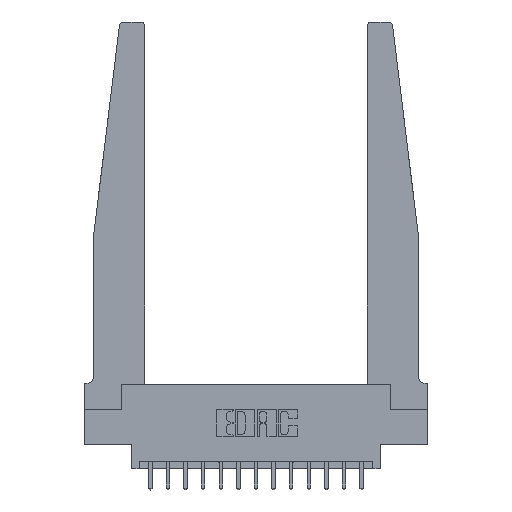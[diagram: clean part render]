
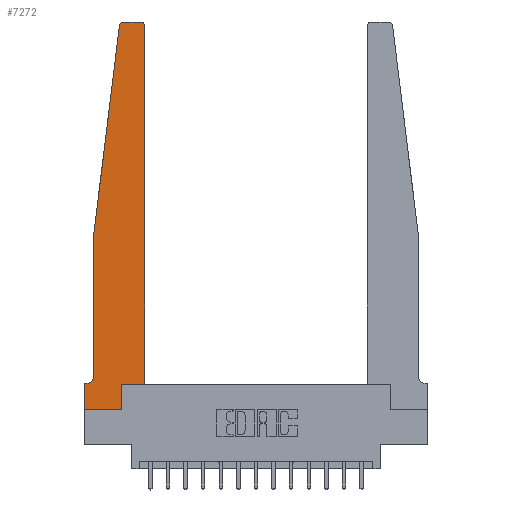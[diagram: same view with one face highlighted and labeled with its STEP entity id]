
A CAD part, top view. The second image highlights one B-rep face of the part: STEP entity #7272.
In plain terms, the highlighted planar face has unit normal (0, 0, 1).
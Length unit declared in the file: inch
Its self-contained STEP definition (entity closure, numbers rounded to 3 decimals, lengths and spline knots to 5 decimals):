
#203 = DIRECTION ( 'NONE',  ( 0., 1., 0. ) ) ;
#871 = CARTESIAN_POINT ( 'NONE',  ( 0.395, 2.75, 0.37 ) ) ;
#1552 = AXIS2_PLACEMENT_3D ( 'NONE', #4527, #13935, #5878 ) ;
#1663 = DIRECTION ( 'NONE',  ( 0., 0., 1. ) ) ;
#1771 = CARTESIAN_POINT ( 'NONE',  ( 0.065, 0.1875, 0.37 ) ) ;
#2200 = CARTESIAN_POINT ( 'NONE',  ( 0.065, 1.25, 0.37 ) ) ;
#2266 = ORIENTED_EDGE ( 'NONE', *, *, #3046, .T. ) ;
#2368 = VERTEX_POINT ( 'NONE', #9925 ) ;
#2550 = LINE ( 'NONE', #16554, #9312 ) ;
#2705 = CIRCLE ( 'NONE', #4445, 0.03 ) ;
#2726 = DIRECTION ( 'NONE',  ( 1., 0., 0. ) ) ;
#2876 = CARTESIAN_POINT ( 'NONE',  ( 0.425, 2.72, 0.37 ) ) ;
#3022 = VERTEX_POINT ( 'NONE', #5765 ) ;
#3046 = EDGE_CURVE ( 'NONE', #10043, #12302, #9291, .T. ) ;
#3104 = DIRECTION ( 'NONE',  ( -1., 0., 0. ) ) ;
#3427 = EDGE_CURVE ( 'NONE', #2368, #12764, #3769, .T. ) ;
#3631 = EDGE_CURVE ( 'NONE', #12302, #16082, #4388, .T. ) ;
#3719 = EDGE_CURVE ( 'NONE', #3022, #17066, #2705, .T. ) ;
#3769 = LINE ( 'NONE', #13399, #14915 ) ;
#3974 = VECTOR ( 'NONE', #3104, 39.37008 ) ;
#3977 = CARTESIAN_POINT ( 'NONE',  ( 0.24675, 2.72367, 0.37 ) ) ;
#4288 = FACE_OUTER_BOUND ( 'NONE', #10441, .T. ) ;
#4388 = LINE ( 'NONE', #1771, #3974 ) ;
#4445 = AXIS2_PLACEMENT_3D ( 'NONE', #14035, #5969, #15380 ) ;
#4527 = CARTESIAN_POINT ( 'NONE',  ( 0.015, 0.2375, 0.37 ) ) ;
#4588 = AXIS2_PLACEMENT_3D ( 'NONE', #9711, #1663, #11053 ) ;
#4644 = LINE ( 'NONE', #16207, #14944 ) ;
#4767 = EDGE_CURVE ( 'NONE', #14170, #13829, #16121, .T. ) ;
#5006 = EDGE_CURVE ( 'NONE', #13829, #3022, #5191, .T. ) ;
#5051 = CARTESIAN_POINT ( 'NONE',  ( 0.2605, 0.18, 0.37 ) ) ;
#5129 = VECTOR ( 'NONE', #5737, 39.37008 ) ;
#5135 = VECTOR ( 'NONE', #5209, 39.37008 ) ;
#5191 = LINE ( 'NONE', #7569, #12761 ) ;
#5209 = DIRECTION ( 'NONE',  ( 0., -1., 0. ) ) ;
#5737 = DIRECTION ( 'NONE',  ( 0., -1., 0. ) ) ;
#5756 = VECTOR ( 'NONE', #10339, 39.37008 ) ;
#5765 = CARTESIAN_POINT ( 'NONE',  ( 0.27653, 2.75, 0.37 ) ) ;
#5878 = DIRECTION ( 'NONE',  ( -1., 0., 0. ) ) ;
#5969 = DIRECTION ( 'NONE',  ( 0., 0., 1. ) ) ;
#6386 = CARTESIAN_POINT ( 'NONE',  ( 0.425, 0.18, 0.37 ) ) ;
#6639 = DIRECTION ( 'NONE',  ( 0., 1., 0. ) ) ;
#6642 = LINE ( 'NONE', #15164, #13374 ) ;
#6911 = VERTEX_POINT ( 'NONE', #13908 ) ;
#7220 = EDGE_CURVE ( 'NONE', #10985, #10043, #12287, .T. ) ;
#7272 = ADVANCED_FACE ( 'NONE', ( #4288 ), #9468, .T. ) ;
#7569 = CARTESIAN_POINT ( 'NONE',  ( 0.25, 2.75, 0.37 ) ) ;
#7962 = ORIENTED_EDGE ( 'NONE', *, *, #3427, .T. ) ;
#8166 = ORIENTED_EDGE ( 'NONE', *, *, #3719, .T. ) ;
#8804 = ORIENTED_EDGE ( 'NONE', *, *, #16212, .T. ) ;
#9107 = CARTESIAN_POINT ( 'NONE',  ( 0.015, 0.1875, 0.37 ) ) ;
#9291 = CIRCLE ( 'NONE', #1552, 0.05 ) ;
#9312 = VECTOR ( 'NONE', #12513, 39.37008 ) ;
#9468 = PLANE ( 'NONE',  #15727 ) ;
#9579 = LINE ( 'NONE', #9816, #5129 ) ;
#9711 = CARTESIAN_POINT ( 'NONE',  ( 0.395, 2.72, 0.37 ) ) ;
#9816 = CARTESIAN_POINT ( 'NONE',  ( 0., 0., 0.37 ) ) ;
#9925 = CARTESIAN_POINT ( 'NONE',  ( 0.2605, 0., 0.37 ) ) ;
#10043 = VERTEX_POINT ( 'NONE', #15081 ) ;
#10288 = DIRECTION ( 'NONE',  ( -1., 0., 0. ) ) ;
#10339 = DIRECTION ( 'NONE',  ( -0.122, -0.992, 0. ) ) ;
#10441 = EDGE_LOOP ( 'NONE', ( #14026, #8166, #11723, #12134, #2266, #13404, #16943, #10689, #7962, #8804, #12351, #12772 ) ) ;
#10689 = ORIENTED_EDGE ( 'NONE', *, *, #14270, .T. ) ;
#10747 = CARTESIAN_POINT ( 'NONE',  ( 0., 0.1875, 0.37 ) ) ;
#10806 = DIRECTION ( 'NONE',  ( 0., 0., 1. ) ) ;
#10985 = VERTEX_POINT ( 'NONE', #2200 ) ;
#11053 = DIRECTION ( 'NONE',  ( 1., 0., 0. ) ) ;
#11723 = ORIENTED_EDGE ( 'NONE', *, *, #12260, .T. ) ;
#12065 = EDGE_CURVE ( 'NONE', #16082, #6911, #9579, .T. ) ;
#12134 = ORIENTED_EDGE ( 'NONE', *, *, #7220, .T. ) ;
#12260 = EDGE_CURVE ( 'NONE', #17066, #10985, #16879, .T. ) ;
#12287 = LINE ( 'NONE', #16057, #5135 ) ;
#12302 = VERTEX_POINT ( 'NONE', #9107 ) ;
#12351 = ORIENTED_EDGE ( 'NONE', *, *, #14098, .T. ) ;
#12513 = DIRECTION ( 'NONE',  ( 1., 0., 0. ) ) ;
#12761 = VECTOR ( 'NONE', #10288, 39.37008 ) ;
#12764 = VERTEX_POINT ( 'NONE', #5051 ) ;
#12772 = ORIENTED_EDGE ( 'NONE', *, *, #4767, .T. ) ;
#13374 = VECTOR ( 'NONE', #16565, 39.37008 ) ;
#13399 = CARTESIAN_POINT ( 'NONE',  ( 0.2605, 0.18, 0.37 ) ) ;
#13404 = ORIENTED_EDGE ( 'NONE', *, *, #3631, .T. ) ;
#13829 = VERTEX_POINT ( 'NONE', #871 ) ;
#13908 = CARTESIAN_POINT ( 'NONE',  ( 0., 0., 0.37 ) ) ;
#13935 = DIRECTION ( 'NONE',  ( 0., 0., -1. ) ) ;
#14026 = ORIENTED_EDGE ( 'NONE', *, *, #5006, .T. ) ;
#14035 = CARTESIAN_POINT ( 'NONE',  ( 0.27653, 2.72, 0.37 ) ) ;
#14098 = EDGE_CURVE ( 'NONE', #14566, #14170, #4644, .T. ) ;
#14170 = VERTEX_POINT ( 'NONE', #2876 ) ;
#14270 = EDGE_CURVE ( 'NONE', #6911, #2368, #2550, .T. ) ;
#14308 = CARTESIAN_POINT ( 'NONE',  ( 0.065, 1.25, 0.37 ) ) ;
#14566 = VERTEX_POINT ( 'NONE', #6386 ) ;
#14915 = VECTOR ( 'NONE', #6639, 39.37008 ) ;
#14944 = VECTOR ( 'NONE', #203, 39.37008 ) ;
#15081 = CARTESIAN_POINT ( 'NONE',  ( 0.065, 0.2375, 0.37 ) ) ;
#15164 = CARTESIAN_POINT ( 'NONE',  ( 0.425, 0.18, 0.37 ) ) ;
#15380 = DIRECTION ( 'NONE',  ( 1., 0., 0. ) ) ;
#15727 = AXIS2_PLACEMENT_3D ( 'NONE', #10747, #10806, #2726 ) ;
#16057 = CARTESIAN_POINT ( 'NONE',  ( 0.065, 1.25, 0.37 ) ) ;
#16082 = VERTEX_POINT ( 'NONE', #16222 ) ;
#16121 = CIRCLE ( 'NONE', #4588, 0.03 ) ;
#16207 = CARTESIAN_POINT ( 'NONE',  ( 0.425, 0.18, 0.37 ) ) ;
#16212 = EDGE_CURVE ( 'NONE', #12764, #14566, #6642, .T. ) ;
#16222 = CARTESIAN_POINT ( 'NONE',  ( 0., 0.1875, 0.37 ) ) ;
#16554 = CARTESIAN_POINT ( 'NONE',  ( 0., 0., 0.37 ) ) ;
#16565 = DIRECTION ( 'NONE',  ( 1., 0., 0. ) ) ;
#16879 = LINE ( 'NONE', #14308, #5756 ) ;
#16943 = ORIENTED_EDGE ( 'NONE', *, *, #12065, .T. ) ;
#17066 = VERTEX_POINT ( 'NONE', #3977 ) ;
